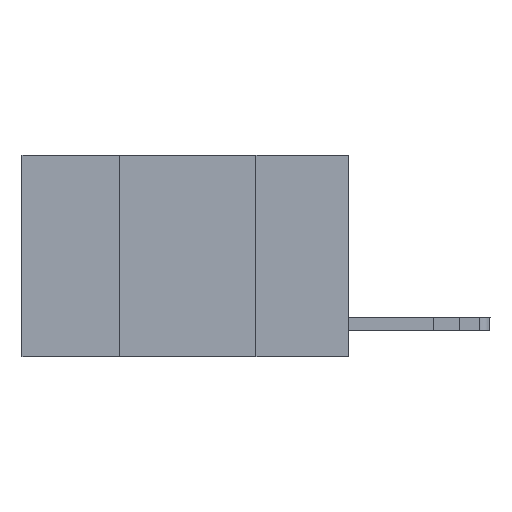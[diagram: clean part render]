
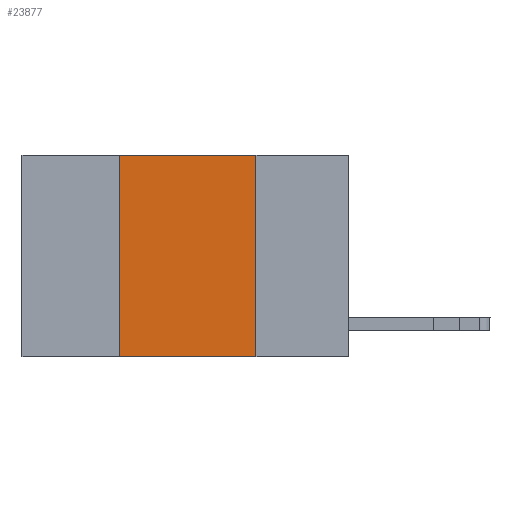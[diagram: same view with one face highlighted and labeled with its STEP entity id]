
A CAD part, left-side view. The second image highlights one B-rep face of the part: STEP entity #23877.
In plain terms, the highlighted planar face has unit normal (-1, 0, 0).
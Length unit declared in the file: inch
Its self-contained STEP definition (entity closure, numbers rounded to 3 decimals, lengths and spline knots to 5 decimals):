
#260 = EDGE_CURVE ( 'NONE', #14812, #3902, #19462, .T. ) ;
#564 = LINE ( 'NONE', #23258, #12991 ) ;
#1991 = CARTESIAN_POINT ( 'NONE',  ( 0., 0.6, 0. ) ) ;
#3105 = EDGE_CURVE ( 'NONE', #19497, #3215, #564, .T. ) ;
#3215 = VERTEX_POINT ( 'NONE', #21731 ) ;
#3598 = CARTESIAN_POINT ( 'NONE',  ( 0., 0.6, -0.37 ) ) ;
#3902 = VERTEX_POINT ( 'NONE', #15985 ) ;
#4361 = DIRECTION ( 'NONE',  ( 0., 0., 1. ) ) ;
#6931 = ORIENTED_EDGE ( 'NONE', *, *, #3105, .F. ) ;
#8508 = FACE_OUTER_BOUND ( 'NONE', #18424, .T. ) ;
#8564 = DIRECTION ( 'NONE',  ( 0., 0., -1. ) ) ;
#8999 = ORIENTED_EDGE ( 'NONE', *, *, #260, .F. ) ;
#9803 = DIRECTION ( 'NONE',  ( 0., -1., 0. ) ) ;
#12393 = EDGE_CURVE ( 'NONE', #19497, #3902, #20041, .T. ) ;
#12428 = CARTESIAN_POINT ( 'NONE',  ( 0., 0.42, -0.37 ) ) ;
#12642 = VECTOR ( 'NONE', #9803, 39.37008 ) ;
#12682 = VECTOR ( 'NONE', #8564, 39.37008 ) ;
#12991 = VECTOR ( 'NONE', #4361, 39.37008 ) ;
#13809 = EDGE_CURVE ( 'NONE', #3215, #14812, #14183, .T. ) ;
#14183 = LINE ( 'NONE', #16229, #23795 ) ;
#14812 = VERTEX_POINT ( 'NONE', #18900 ) ;
#14954 = CARTESIAN_POINT ( 'NONE',  ( 0., 0.17, 0. ) ) ;
#15985 = CARTESIAN_POINT ( 'NONE',  ( 0., 0.17, -0.37 ) ) ;
#16229 = CARTESIAN_POINT ( 'NONE',  ( 0., 0.6, 0. ) ) ;
#18285 = ORIENTED_EDGE ( 'NONE', *, *, #12393, .T. ) ;
#18337 = DIRECTION ( 'NONE',  ( 0., 0., -1. ) ) ;
#18424 = EDGE_LOOP ( 'NONE', ( #8999, #20358, #6931, #18285 ) ) ;
#18900 = CARTESIAN_POINT ( 'NONE',  ( 0., 0.17, 0. ) ) ;
#19462 = LINE ( 'NONE', #14954, #12682 ) ;
#19497 = VERTEX_POINT ( 'NONE', #12428 ) ;
#20041 = LINE ( 'NONE', #3598, #12642 ) ;
#20335 = DIRECTION ( 'NONE',  ( 0., -1., 0. ) ) ;
#20358 = ORIENTED_EDGE ( 'NONE', *, *, #13809, .F. ) ;
#20772 = DIRECTION ( 'NONE',  ( 1., 0., 0. ) ) ;
#21731 = CARTESIAN_POINT ( 'NONE',  ( 0., 0.42, 0. ) ) ;
#21767 = AXIS2_PLACEMENT_3D ( 'NONE', #1991, #20772, #18337 ) ;
#22545 = PLANE ( 'NONE',  #21767 ) ;
#23258 = CARTESIAN_POINT ( 'NONE',  ( 0., 0.42, 0. ) ) ;
#23795 = VECTOR ( 'NONE', #20335, 39.37008 ) ;
#23877 = ADVANCED_FACE ( 'NONE', ( #8508 ), #22545, .F. ) ;
